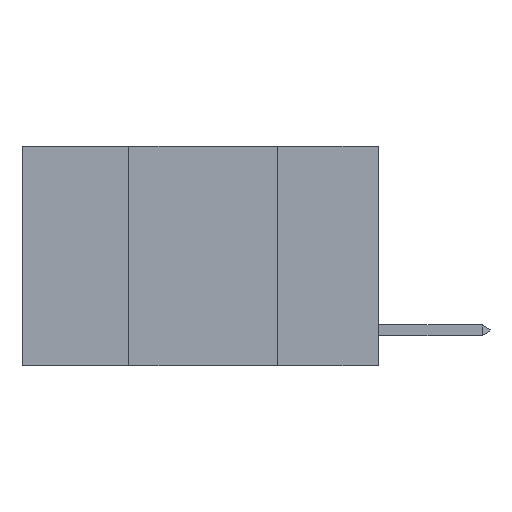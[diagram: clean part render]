
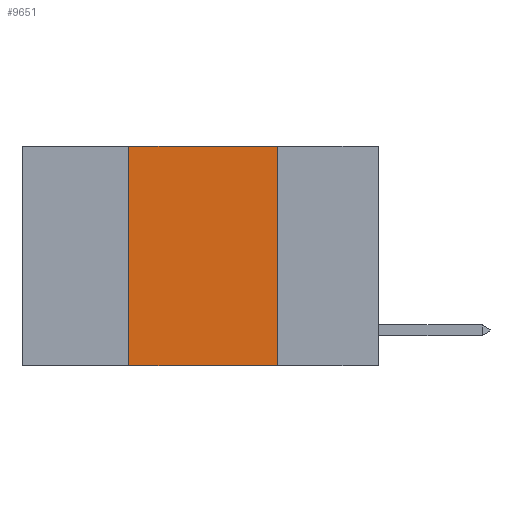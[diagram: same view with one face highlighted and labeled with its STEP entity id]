
A CAD part, left-side view. The second image highlights one B-rep face of the part: STEP entity #9651.
In plain terms, the highlighted planar face has unit normal (-1, 0, 0).
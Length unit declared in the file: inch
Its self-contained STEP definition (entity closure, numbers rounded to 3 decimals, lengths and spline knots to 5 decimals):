
#287 = EDGE_CURVE ( 'NONE', #6650, #7168, #6590, .T. ) ;
#2049 = DIRECTION ( 'NONE',  ( 0., -1., 0. ) ) ;
#2360 = CARTESIAN_POINT ( 'NONE',  ( 0., 0.17, 0. ) ) ;
#2414 = CARTESIAN_POINT ( 'NONE',  ( 0., 0.42, 0. ) ) ;
#2926 = PLANE ( 'NONE',  #9251 ) ;
#3350 = ORIENTED_EDGE ( 'NONE', *, *, #287, .F. ) ;
#3686 = FACE_OUTER_BOUND ( 'NONE', #8813, .T. ) ;
#3752 = VECTOR ( 'NONE', #8769, 39.37008 ) ;
#3837 = DIRECTION ( 'NONE',  ( 0., 0., -1. ) ) ;
#4054 = CARTESIAN_POINT ( 'NONE',  ( 0., 0.6, 0. ) ) ;
#4729 = CARTESIAN_POINT ( 'NONE',  ( 0., 0.6, -0.37 ) ) ;
#5008 = VERTEX_POINT ( 'NONE', #2414 ) ;
#5031 = LINE ( 'NONE', #4054, #5289 ) ;
#5289 = VECTOR ( 'NONE', #7482, 39.37008 ) ;
#5348 = CARTESIAN_POINT ( 'NONE',  ( 0., 0.17, 0. ) ) ;
#5669 = ORIENTED_EDGE ( 'NONE', *, *, #10469, .F. ) ;
#5764 = VERTEX_POINT ( 'NONE', #10263 ) ;
#5924 = ORIENTED_EDGE ( 'NONE', *, *, #10454, .F. ) ;
#6535 = VECTOR ( 'NONE', #2049, 39.37008 ) ;
#6590 = LINE ( 'NONE', #5348, #3752 ) ;
#6650 = VERTEX_POINT ( 'NONE', #2360 ) ;
#7168 = VERTEX_POINT ( 'NONE', #8306 ) ;
#7482 = DIRECTION ( 'NONE',  ( 0., -1., 0. ) ) ;
#8295 = EDGE_CURVE ( 'NONE', #5764, #7168, #11186, .T. ) ;
#8306 = CARTESIAN_POINT ( 'NONE',  ( 0., 0.17, -0.37 ) ) ;
#8769 = DIRECTION ( 'NONE',  ( 0., 0., -1. ) ) ;
#8813 = EDGE_LOOP ( 'NONE', ( #3350, #5669, #5924, #10881 ) ) ;
#9037 = DIRECTION ( 'NONE',  ( 1., 0., 0. ) ) ;
#9219 = DIRECTION ( 'NONE',  ( 0., 0., 1. ) ) ;
#9251 = AXIS2_PLACEMENT_3D ( 'NONE', #10561, #9037, #3837 ) ;
#9346 = VECTOR ( 'NONE', #9219, 39.37008 ) ;
#9592 = LINE ( 'NONE', #10752, #9346 ) ;
#9651 = ADVANCED_FACE ( 'NONE', ( #3686 ), #2926, .F. ) ;
#10263 = CARTESIAN_POINT ( 'NONE',  ( 0., 0.42, -0.37 ) ) ;
#10454 = EDGE_CURVE ( 'NONE', #5764, #5008, #9592, .T. ) ;
#10469 = EDGE_CURVE ( 'NONE', #5008, #6650, #5031, .T. ) ;
#10561 = CARTESIAN_POINT ( 'NONE',  ( 0., 0.6, 0. ) ) ;
#10752 = CARTESIAN_POINT ( 'NONE',  ( 0., 0.42, 0. ) ) ;
#10881 = ORIENTED_EDGE ( 'NONE', *, *, #8295, .T. ) ;
#11186 = LINE ( 'NONE', #4729, #6535 ) ;
